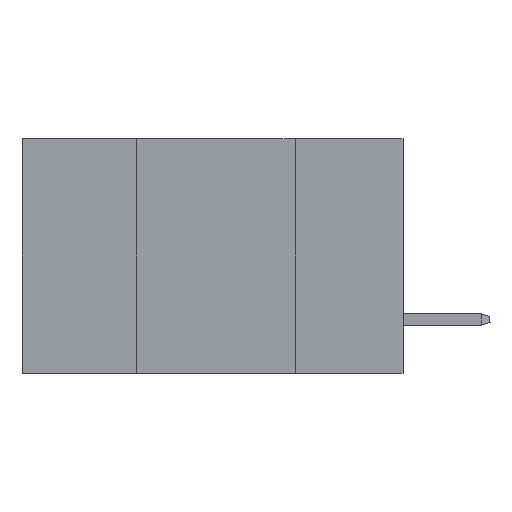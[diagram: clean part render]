
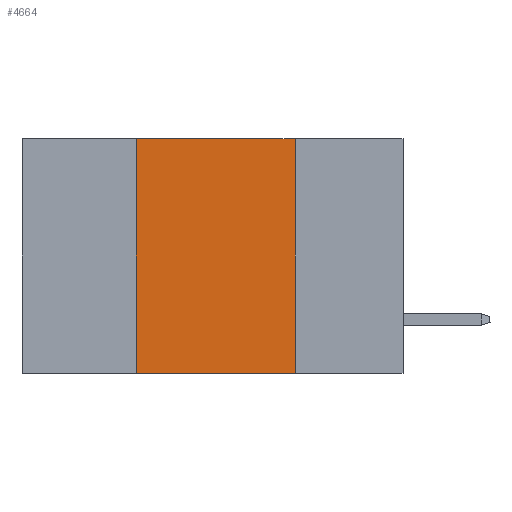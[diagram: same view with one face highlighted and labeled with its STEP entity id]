
A CAD part, left-side view. The second image highlights one B-rep face of the part: STEP entity #4664.
In plain terms, the highlighted planar face has unit normal (-1, 0, 0).
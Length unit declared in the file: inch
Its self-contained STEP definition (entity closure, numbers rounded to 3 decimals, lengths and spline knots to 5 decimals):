
#591 = EDGE_CURVE ( 'NONE', #5619, #13302, #5777, .T. ) ;
#851 = DIRECTION ( 'NONE',  ( 0., -1., 0. ) ) ;
#1011 = PLANE ( 'NONE',  #3982 ) ;
#2172 = ORIENTED_EDGE ( 'NONE', *, *, #9060, .T. ) ;
#2193 = LINE ( 'NONE', #9405, #13636 ) ;
#2597 = DIRECTION ( 'NONE',  ( 1., 0., 0. ) ) ;
#2925 = EDGE_CURVE ( 'NONE', #12554, #19131, #2193, .T. ) ;
#3693 = FACE_OUTER_BOUND ( 'NONE', #7517, .T. ) ;
#3859 = CARTESIAN_POINT ( 'NONE',  ( 0., 0.42, 0. ) ) ;
#3982 = AXIS2_PLACEMENT_3D ( 'NONE', #19049, #2597, #7214 ) ;
#3990 = CARTESIAN_POINT ( 'NONE',  ( 0., 0.6, 0. ) ) ;
#4664 = ADVANCED_FACE ( 'NONE', ( #3693 ), #1011, .F. ) ;
#4967 = VECTOR ( 'NONE', #5074, 39.37008 ) ;
#4978 = DIRECTION ( 'NONE',  ( 0., 0., -1. ) ) ;
#5074 = DIRECTION ( 'NONE',  ( 0., -1., 0. ) ) ;
#5619 = VERTEX_POINT ( 'NONE', #17702 ) ;
#5777 = LINE ( 'NONE', #17621, #18516 ) ;
#6543 = CARTESIAN_POINT ( 'NONE',  ( 0., 0.17, 0. ) ) ;
#6741 = LINE ( 'NONE', #3990, #4967 ) ;
#7214 = DIRECTION ( 'NONE',  ( 0., 0., -1. ) ) ;
#7517 = EDGE_LOOP ( 'NONE', ( #18300, #8379, #11636, #2172 ) ) ;
#8336 = CARTESIAN_POINT ( 'NONE',  ( 0., 0.6, -0.37 ) ) ;
#8379 = ORIENTED_EDGE ( 'NONE', *, *, #17562, .F. ) ;
#8771 = VECTOR ( 'NONE', #851, 39.37008 ) ;
#9060 = EDGE_CURVE ( 'NONE', #5619, #19131, #9837, .T. ) ;
#9405 = CARTESIAN_POINT ( 'NONE',  ( 0., 0.17, 0. ) ) ;
#9837 = LINE ( 'NONE', #8336, #8771 ) ;
#10132 = DIRECTION ( 'NONE',  ( 0., 0., 1. ) ) ;
#11636 = ORIENTED_EDGE ( 'NONE', *, *, #591, .F. ) ;
#12554 = VERTEX_POINT ( 'NONE', #6543 ) ;
#13302 = VERTEX_POINT ( 'NONE', #3859 ) ;
#13636 = VECTOR ( 'NONE', #4978, 39.37008 ) ;
#17562 = EDGE_CURVE ( 'NONE', #13302, #12554, #6741, .T. ) ;
#17621 = CARTESIAN_POINT ( 'NONE',  ( 0., 0.42, 0. ) ) ;
#17702 = CARTESIAN_POINT ( 'NONE',  ( 0., 0.42, -0.37 ) ) ;
#18300 = ORIENTED_EDGE ( 'NONE', *, *, #2925, .F. ) ;
#18516 = VECTOR ( 'NONE', #10132, 39.37008 ) ;
#19049 = CARTESIAN_POINT ( 'NONE',  ( 0., 0.6, 0. ) ) ;
#19081 = CARTESIAN_POINT ( 'NONE',  ( 0., 0.17, -0.37 ) ) ;
#19131 = VERTEX_POINT ( 'NONE', #19081 ) ;
